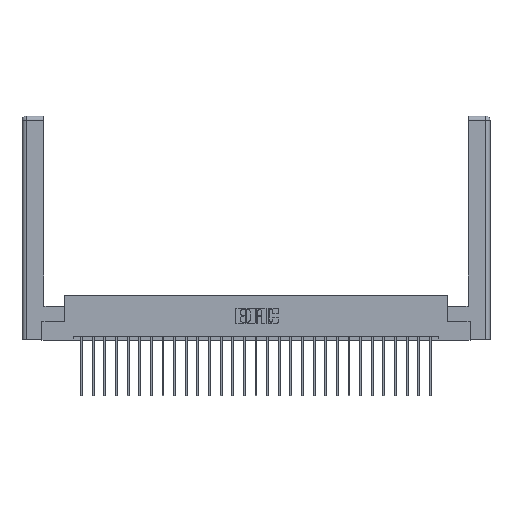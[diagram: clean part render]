
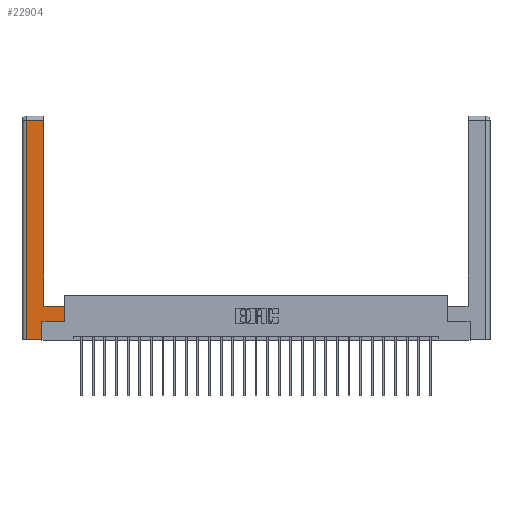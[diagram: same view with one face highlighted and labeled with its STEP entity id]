
A CAD part, top view. The second image highlights one B-rep face of the part: STEP entity #22904.
In plain terms, the highlighted planar face has unit normal (0, 0, 1).
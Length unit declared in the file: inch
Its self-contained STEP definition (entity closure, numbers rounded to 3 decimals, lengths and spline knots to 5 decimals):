
#820 = ORIENTED_EDGE ( 'NONE', *, *, #17177, .T. ) ;
#1296 = VECTOR ( 'NONE', #13802, 39.37008 ) ;
#1301 = DIRECTION ( 'NONE',  ( 0., 1., 0. ) ) ;
#1549 = DIRECTION ( 'NONE',  ( -1., 0., 0. ) ) ;
#1764 = VERTEX_POINT ( 'NONE', #22073 ) ;
#2173 = CARTESIAN_POINT ( 'NONE',  ( 0.265, 0., 0. ) ) ;
#2238 = DIRECTION ( 'NONE',  ( 1., 0., 0. ) ) ;
#4088 = ORIENTED_EDGE ( 'NONE', *, *, #24729, .T. ) ;
#4508 = DIRECTION ( 'NONE',  ( 0., -1., 0. ) ) ;
#4674 = VECTOR ( 'NONE', #22223, 39.37008 ) ;
#5487 = ORIENTED_EDGE ( 'NONE', *, *, #12743, .T. ) ;
#5702 = CARTESIAN_POINT ( 'NONE',  ( 0.565, 0.45, 0. ) ) ;
#6075 = EDGE_CURVE ( 'NONE', #19851, #11566, #12928, .T. ) ;
#6203 = CARTESIAN_POINT ( 'NONE',  ( 0.265, 0., 0. ) ) ;
#7432 = AXIS2_PLACEMENT_3D ( 'NONE', #9769, #14007, #24924 ) ;
#7876 = VECTOR ( 'NONE', #2238, 39.37008 ) ;
#8783 = EDGE_LOOP ( 'NONE', ( #4088, #25465, #23738, #5487, #14116, #820, #17496, #23106 ) ) ;
#9085 = VERTEX_POINT ( 'NONE', #20974 ) ;
#9188 = EDGE_CURVE ( 'NONE', #1764, #19840, #16910, .T. ) ;
#9769 = CARTESIAN_POINT ( 'NONE',  ( 0., 0., 0. ) ) ;
#11566 = VERTEX_POINT ( 'NONE', #22154 ) ;
#11993 = LINE ( 'NONE', #24317, #7876 ) ;
#11998 = VERTEX_POINT ( 'NONE', #28017 ) ;
#12743 = EDGE_CURVE ( 'NONE', #14051, #19851, #20032, .T. ) ;
#12829 = EDGE_CURVE ( 'NONE', #11998, #9085, #22746, .T. ) ;
#12928 = LINE ( 'NONE', #15678, #13641 ) ;
#12957 = CARTESIAN_POINT ( 'NONE',  ( 0.565, 0.45, 0. ) ) ;
#13201 = VECTOR ( 'NONE', #1549, 39.37008 ) ;
#13212 = CARTESIAN_POINT ( 'NONE',  ( 0.0615, 0., 0. ) ) ;
#13601 = DIRECTION ( 'NONE',  ( 0., 1., 0. ) ) ;
#13641 = VECTOR ( 'NONE', #13601, 39.37008 ) ;
#13802 = DIRECTION ( 'NONE',  ( 0., 1., 0. ) ) ;
#13967 = VERTEX_POINT ( 'NONE', #19571 ) ;
#14007 = DIRECTION ( 'NONE',  ( 0., 0., -1. ) ) ;
#14051 = VERTEX_POINT ( 'NONE', #17678 ) ;
#14116 = ORIENTED_EDGE ( 'NONE', *, *, #6075, .T. ) ;
#14237 = LINE ( 'NONE', #26181, #1296 ) ;
#15355 = FACE_OUTER_BOUND ( 'NONE', #8783, .T. ) ;
#15382 = CARTESIAN_POINT ( 'NONE',  ( 0.0615, 2.94, 0. ) ) ;
#15678 = CARTESIAN_POINT ( 'NONE',  ( 0.265, 0.245, 0. ) ) ;
#16304 = VECTOR ( 'NONE', #21470, 39.37008 ) ;
#16569 = VECTOR ( 'NONE', #1301, 39.37008 ) ;
#16734 = EDGE_CURVE ( 'NONE', #9085, #14051, #16782, .T. ) ;
#16769 = CARTESIAN_POINT ( 'NONE',  ( 0.295, 0.45, 0. ) ) ;
#16782 = LINE ( 'NONE', #13212, #23916 ) ;
#16910 = LINE ( 'NONE', #5702, #16569 ) ;
#17177 = EDGE_CURVE ( 'NONE', #11566, #1764, #11993, .T. ) ;
#17496 = ORIENTED_EDGE ( 'NONE', *, *, #9188, .T. ) ;
#17678 = CARTESIAN_POINT ( 'NONE',  ( 0.0615, 0., 0. ) ) ;
#17998 = LINE ( 'NONE', #16769, #13201 ) ;
#19571 = CARTESIAN_POINT ( 'NONE',  ( 0.295, 0.45, 0. ) ) ;
#19840 = VERTEX_POINT ( 'NONE', #12957 ) ;
#19851 = VERTEX_POINT ( 'NONE', #2173 ) ;
#20032 = LINE ( 'NONE', #6203, #16304 ) ;
#20974 = CARTESIAN_POINT ( 'NONE',  ( 0.0615, 2.94, 0. ) ) ;
#21470 = DIRECTION ( 'NONE',  ( 1., 0., 0. ) ) ;
#22073 = CARTESIAN_POINT ( 'NONE',  ( 0.565, 0.245, 0. ) ) ;
#22154 = CARTESIAN_POINT ( 'NONE',  ( 0.265, 0.245, 0. ) ) ;
#22223 = DIRECTION ( 'NONE',  ( -1., 0., 0. ) ) ;
#22746 = LINE ( 'NONE', #15382, #4674 ) ;
#22904 = ADVANCED_FACE ( 'NONE', ( #15355 ), #27217, .F. ) ;
#23106 = ORIENTED_EDGE ( 'NONE', *, *, #27547, .T. ) ;
#23738 = ORIENTED_EDGE ( 'NONE', *, *, #16734, .T. ) ;
#23916 = VECTOR ( 'NONE', #4508, 39.37008 ) ;
#24317 = CARTESIAN_POINT ( 'NONE',  ( 0.565, 0.245, 0. ) ) ;
#24729 = EDGE_CURVE ( 'NONE', #13967, #11998, #14237, .T. ) ;
#24924 = DIRECTION ( 'NONE',  ( -1., 0., 0. ) ) ;
#25465 = ORIENTED_EDGE ( 'NONE', *, *, #12829, .T. ) ;
#26181 = CARTESIAN_POINT ( 'NONE',  ( 0.295, 3., 0. ) ) ;
#27217 = PLANE ( 'NONE',  #7432 ) ;
#27547 = EDGE_CURVE ( 'NONE', #19840, #13967, #17998, .T. ) ;
#28017 = CARTESIAN_POINT ( 'NONE',  ( 0.295, 2.94, 0. ) ) ;
